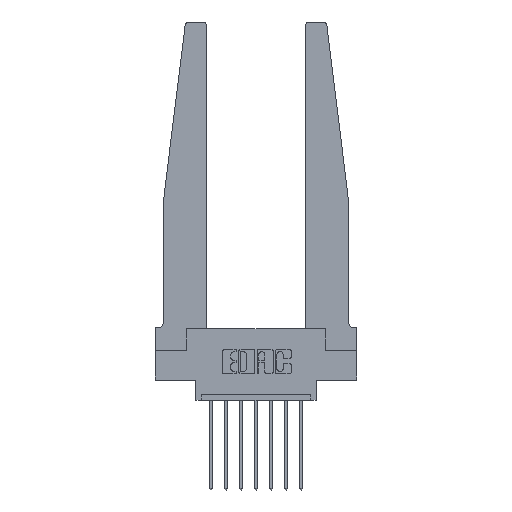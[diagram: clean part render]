
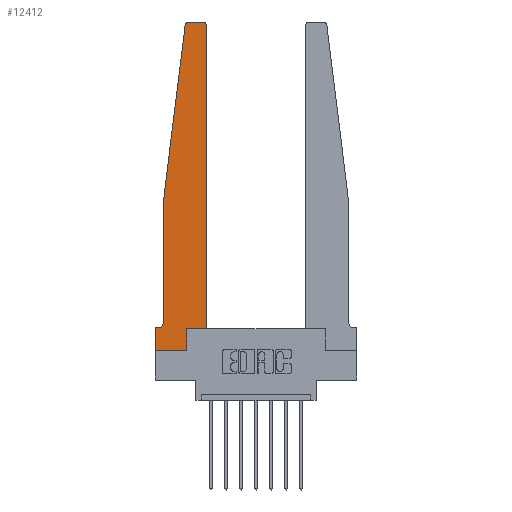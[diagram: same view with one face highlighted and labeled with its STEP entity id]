
A CAD part, top view. The second image highlights one B-rep face of the part: STEP entity #12412.
In plain terms, the highlighted planar face has unit normal (0, 0, 1).
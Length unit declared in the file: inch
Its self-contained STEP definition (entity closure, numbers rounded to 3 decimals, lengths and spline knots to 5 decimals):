
#426 = LINE ( 'NONE', #808, #7490 ) ;
#477 = DIRECTION ( 'NONE',  ( 0., 0., 1. ) ) ;
#501 = DIRECTION ( 'NONE',  ( 0., 0., 1. ) ) ;
#572 = ORIENTED_EDGE ( 'NONE', *, *, #1052, .T. ) ;
#597 = CARTESIAN_POINT ( 'NONE',  ( 0.27653, 2.72, 0.37 ) ) ;
#631 = VERTEX_POINT ( 'NONE', #6371 ) ;
#664 = VECTOR ( 'NONE', #5302, 39.37008 ) ;
#754 = FACE_OUTER_BOUND ( 'NONE', #10735, .T. ) ;
#808 = CARTESIAN_POINT ( 'NONE',  ( 0.065, 0.1875, 0.37 ) ) ;
#918 = VERTEX_POINT ( 'NONE', #7438 ) ;
#957 = VERTEX_POINT ( 'NONE', #7911 ) ;
#976 = EDGE_CURVE ( 'NONE', #957, #11595, #10034, .T. ) ;
#1015 = VECTOR ( 'NONE', #4760, 39.37008 ) ;
#1052 = EDGE_CURVE ( 'NONE', #11520, #9317, #5002, .T. ) ;
#1056 = DIRECTION ( 'NONE',  ( 0., 0., 1. ) ) ;
#1082 = LINE ( 'NONE', #11522, #2949 ) ;
#1195 = AXIS2_PLACEMENT_3D ( 'NONE', #13417, #477, #5825 ) ;
#1692 = LINE ( 'NONE', #3303, #664 ) ;
#2160 = CIRCLE ( 'NONE', #5503, 0.05 ) ;
#2177 = VECTOR ( 'NONE', #11769, 39.37008 ) ;
#2313 = CARTESIAN_POINT ( 'NONE',  ( 0.395, 2.72, 0.37 ) ) ;
#2390 = CARTESIAN_POINT ( 'NONE',  ( 0.2605, 0.18, 0.37 ) ) ;
#2503 = VECTOR ( 'NONE', #9303, 39.37008 ) ;
#2664 = LINE ( 'NONE', #7521, #9044 ) ;
#2771 = EDGE_CURVE ( 'NONE', #9203, #11520, #1082, .T. ) ;
#2871 = CARTESIAN_POINT ( 'NONE',  ( 0.2605, 0., 0.37 ) ) ;
#2949 = VECTOR ( 'NONE', #12558, 39.37008 ) ;
#3303 = CARTESIAN_POINT ( 'NONE',  ( 0., 0., 0.37 ) ) ;
#3347 = DIRECTION ( 'NONE',  ( 0., 0., -1. ) ) ;
#3715 = CIRCLE ( 'NONE', #7449, 0.03 ) ;
#3985 = CARTESIAN_POINT ( 'NONE',  ( 0., 0., 0.37 ) ) ;
#4316 = EDGE_CURVE ( 'NONE', #10313, #5895, #10457, .T. ) ;
#4667 = CARTESIAN_POINT ( 'NONE',  ( 0.25, 2.75, 0.37 ) ) ;
#4760 = DIRECTION ( 'NONE',  ( -1., 0., 0. ) ) ;
#5002 = LINE ( 'NONE', #5559, #8187 ) ;
#5302 = DIRECTION ( 'NONE',  ( 0., -1., 0. ) ) ;
#5386 = EDGE_CURVE ( 'NONE', #5895, #8397, #9113, .T. ) ;
#5503 = AXIS2_PLACEMENT_3D ( 'NONE', #13091, #3347, #10992 ) ;
#5559 = CARTESIAN_POINT ( 'NONE',  ( 0.065, 1.25, 0.37 ) ) ;
#5561 = ORIENTED_EDGE ( 'NONE', *, *, #11335, .T. ) ;
#5565 = VERTEX_POINT ( 'NONE', #9318 ) ;
#5825 = DIRECTION ( 'NONE',  ( 1., 0., 0. ) ) ;
#5895 = VERTEX_POINT ( 'NONE', #9010 ) ;
#5920 = CARTESIAN_POINT ( 'NONE',  ( 0.065, 0.2375, 0.37 ) ) ;
#5993 = DIRECTION ( 'NONE',  ( 1., 0., 0. ) ) ;
#6031 = EDGE_CURVE ( 'NONE', #918, #957, #1692, .T. ) ;
#6215 = LINE ( 'NONE', #9012, #9888 ) ;
#6264 = ORIENTED_EDGE ( 'NONE', *, *, #11829, .T. ) ;
#6371 = CARTESIAN_POINT ( 'NONE',  ( 0.015, 0.1875, 0.37 ) ) ;
#6396 = EDGE_CURVE ( 'NONE', #11595, #8634, #11459, .T. ) ;
#6665 = DIRECTION ( 'NONE',  ( 1., 0., 0. ) ) ;
#7406 = DIRECTION ( 'NONE',  ( -1., 0., 0. ) ) ;
#7438 = CARTESIAN_POINT ( 'NONE',  ( 0., 0.1875, 0.37 ) ) ;
#7449 = AXIS2_PLACEMENT_3D ( 'NONE', #597, #501, #5993 ) ;
#7490 = VECTOR ( 'NONE', #7406, 39.37008 ) ;
#7521 = CARTESIAN_POINT ( 'NONE',  ( 0.425, 0.18, 0.37 ) ) ;
#7566 = DIRECTION ( 'NONE',  ( 1., 0., 0. ) ) ;
#7614 = DIRECTION ( 'NONE',  ( 0., -1., 0. ) ) ;
#7755 = ORIENTED_EDGE ( 'NONE', *, *, #11705, .T. ) ;
#7911 = CARTESIAN_POINT ( 'NONE',  ( 0., 0., 0.37 ) ) ;
#8019 = CARTESIAN_POINT ( 'NONE',  ( 0.425, 2.72, 0.37 ) ) ;
#8091 = ORIENTED_EDGE ( 'NONE', *, *, #6396, .T. ) ;
#8187 = VECTOR ( 'NONE', #7614, 39.37008 ) ;
#8298 = CARTESIAN_POINT ( 'NONE',  ( 0.27653, 2.75, 0.37 ) ) ;
#8397 = VERTEX_POINT ( 'NONE', #8298 ) ;
#8634 = VERTEX_POINT ( 'NONE', #2390 ) ;
#8925 = DIRECTION ( 'NONE',  ( 0., 1., 0. ) ) ;
#8948 = PLANE ( 'NONE',  #1195 ) ;
#9010 = CARTESIAN_POINT ( 'NONE',  ( 0.395, 2.75, 0.37 ) ) ;
#9012 = CARTESIAN_POINT ( 'NONE',  ( 0.425, 0.18, 0.37 ) ) ;
#9044 = VECTOR ( 'NONE', #7566, 39.37008 ) ;
#9113 = LINE ( 'NONE', #4667, #1015 ) ;
#9158 = ORIENTED_EDGE ( 'NONE', *, *, #6031, .T. ) ;
#9203 = VERTEX_POINT ( 'NONE', #10879 ) ;
#9303 = DIRECTION ( 'NONE',  ( 1., 0., 0. ) ) ;
#9317 = VERTEX_POINT ( 'NONE', #5920 ) ;
#9318 = CARTESIAN_POINT ( 'NONE',  ( 0.425, 0.18, 0.37 ) ) ;
#9888 = VECTOR ( 'NONE', #8925, 39.37008 ) ;
#10034 = LINE ( 'NONE', #3985, #2503 ) ;
#10313 = VERTEX_POINT ( 'NONE', #8019 ) ;
#10457 = CIRCLE ( 'NONE', #12911, 0.03 ) ;
#10576 = ORIENTED_EDGE ( 'NONE', *, *, #5386, .T. ) ;
#10600 = CARTESIAN_POINT ( 'NONE',  ( 0.2605, 0.18, 0.37 ) ) ;
#10735 = EDGE_LOOP ( 'NONE', ( #10576, #5561, #13775, #572, #7755, #11187, #9158, #12677, #8091, #11213, #6264, #10742 ) ) ;
#10742 = ORIENTED_EDGE ( 'NONE', *, *, #4316, .T. ) ;
#10879 = CARTESIAN_POINT ( 'NONE',  ( 0.24675, 2.72367, 0.37 ) ) ;
#10992 = DIRECTION ( 'NONE',  ( -1., 0., 0. ) ) ;
#11187 = ORIENTED_EDGE ( 'NONE', *, *, #13248, .T. ) ;
#11213 = ORIENTED_EDGE ( 'NONE', *, *, #12203, .T. ) ;
#11335 = EDGE_CURVE ( 'NONE', #8397, #9203, #3715, .T. ) ;
#11459 = LINE ( 'NONE', #10600, #2177 ) ;
#11520 = VERTEX_POINT ( 'NONE', #13711 ) ;
#11522 = CARTESIAN_POINT ( 'NONE',  ( 0.065, 1.25, 0.37 ) ) ;
#11595 = VERTEX_POINT ( 'NONE', #2871 ) ;
#11705 = EDGE_CURVE ( 'NONE', #9317, #631, #2160, .T. ) ;
#11769 = DIRECTION ( 'NONE',  ( 0., 1., 0. ) ) ;
#11829 = EDGE_CURVE ( 'NONE', #5565, #10313, #6215, .T. ) ;
#12203 = EDGE_CURVE ( 'NONE', #8634, #5565, #2664, .T. ) ;
#12412 = ADVANCED_FACE ( 'NONE', ( #754 ), #8948, .T. ) ;
#12558 = DIRECTION ( 'NONE',  ( -0.122, -0.992, 0. ) ) ;
#12677 = ORIENTED_EDGE ( 'NONE', *, *, #976, .T. ) ;
#12911 = AXIS2_PLACEMENT_3D ( 'NONE', #2313, #1056, #6665 ) ;
#13091 = CARTESIAN_POINT ( 'NONE',  ( 0.015, 0.2375, 0.37 ) ) ;
#13248 = EDGE_CURVE ( 'NONE', #631, #918, #426, .T. ) ;
#13417 = CARTESIAN_POINT ( 'NONE',  ( 0., 0.1875, 0.37 ) ) ;
#13711 = CARTESIAN_POINT ( 'NONE',  ( 0.065, 1.25, 0.37 ) ) ;
#13775 = ORIENTED_EDGE ( 'NONE', *, *, #2771, .T. ) ;
